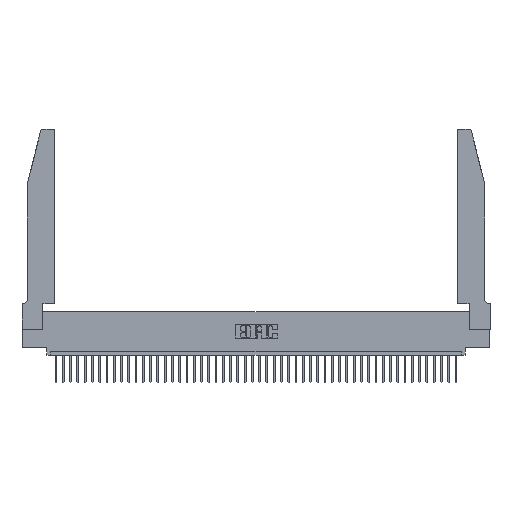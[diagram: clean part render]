
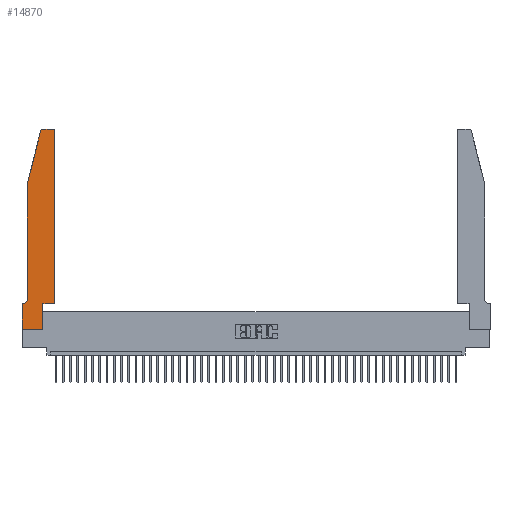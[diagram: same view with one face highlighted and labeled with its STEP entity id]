
A CAD part, top view. The second image highlights one B-rep face of the part: STEP entity #14870.
In plain terms, the highlighted planar face has unit normal (0, 0, 1).
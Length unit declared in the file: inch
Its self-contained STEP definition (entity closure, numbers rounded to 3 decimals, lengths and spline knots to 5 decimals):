
#922 = DIRECTION ( 'NONE',  ( 1., 0., 0. ) ) ;
#1242 = VERTEX_POINT ( 'NONE', #12942 ) ;
#1576 = DIRECTION ( 'NONE',  ( -1., 0., 0. ) ) ;
#1824 = VERTEX_POINT ( 'NONE', #16628 ) ;
#2136 = DIRECTION ( 'NONE',  ( -1., 0., 0. ) ) ;
#3395 = CIRCLE ( 'NONE', #24986, 0.03 ) ;
#4160 = ORIENTED_EDGE ( 'NONE', *, *, #15259, .T. ) ;
#4595 = LINE ( 'NONE', #15943, #15467 ) ;
#4754 = CARTESIAN_POINT ( 'NONE',  ( 0., 0.35, 0.37 ) ) ;
#4789 = EDGE_CURVE ( 'NONE', #6504, #27034, #36625, .T. ) ;
#5355 = ORIENTED_EDGE ( 'NONE', *, *, #10727, .T. ) ;
#5375 = VERTEX_POINT ( 'NONE', #40524 ) ;
#6130 = CARTESIAN_POINT ( 'NONE',  ( 0.0055, 0.42, 0.37 ) ) ;
#6171 = DIRECTION ( 'NONE',  ( 0., 1., 0. ) ) ;
#6495 = VECTOR ( 'NONE', #34825, 39.37008 ) ;
#6504 = VERTEX_POINT ( 'NONE', #4754 ) ;
#6997 = VERTEX_POINT ( 'NONE', #44194 ) ;
#7926 = EDGE_CURVE ( 'NONE', #5375, #38306, #26969, .T. ) ;
#9724 = CARTESIAN_POINT ( 'NONE',  ( 0., 0., 0.37 ) ) ;
#10621 = ORIENTED_EDGE ( 'NONE', *, *, #13284, .T. ) ;
#10727 = EDGE_CURVE ( 'NONE', #31694, #42694, #28785, .T. ) ;
#10803 = ORIENTED_EDGE ( 'NONE', *, *, #26341, .T. ) ;
#10925 = EDGE_CURVE ( 'NONE', #42694, #29869, #11331, .T. ) ;
#11331 = LINE ( 'NONE', #14977, #44713 ) ;
#11994 = AXIS2_PLACEMENT_3D ( 'NONE', #6130, #34358, #1576 ) ;
#12942 = CARTESIAN_POINT ( 'NONE',  ( 0.2865, 0., 0.37 ) ) ;
#13284 = EDGE_CURVE ( 'NONE', #20103, #5375, #24508, .T. ) ;
#14694 = VECTOR ( 'NONE', #44837, 39.37008 ) ;
#14740 = EDGE_CURVE ( 'NONE', #1242, #40147, #40765, .T. ) ;
#14870 = ADVANCED_FACE ( 'NONE', ( #26552 ), #24962, .T. ) ;
#14977 = CARTESIAN_POINT ( 'NONE',  ( 0.0755, 2., 0.37 ) ) ;
#15259 = EDGE_CURVE ( 'NONE', #27034, #1242, #40723, .T. ) ;
#15467 = VECTOR ( 'NONE', #23313, 39.37008 ) ;
#15488 = EDGE_CURVE ( 'NONE', #40147, #6997, #4595, .T. ) ;
#15943 = CARTESIAN_POINT ( 'NONE',  ( 0.4505, 0.35, 0.37 ) ) ;
#15975 = EDGE_LOOP ( 'NONE', ( #27805, #43039, #5355, #23073, #16473, #10803, #36767, #4160, #39724, #18869, #16064, #10621 ) ) ;
#16064 = ORIENTED_EDGE ( 'NONE', *, *, #36062, .T. ) ;
#16112 = CARTESIAN_POINT ( 'NONE',  ( 0.0755, 0.35, 0.37 ) ) ;
#16473 = ORIENTED_EDGE ( 'NONE', *, *, #17511, .T. ) ;
#16628 = CARTESIAN_POINT ( 'NONE',  ( 0.0055, 0.35, 0.37 ) ) ;
#16891 = AXIS2_PLACEMENT_3D ( 'NONE', #42460, #26202, #22196 ) ;
#17511 = EDGE_CURVE ( 'NONE', #29869, #1824, #23569, .T. ) ;
#18200 = DIRECTION ( 'NONE',  ( 1., 0., 0. ) ) ;
#18372 = CARTESIAN_POINT ( 'NONE',  ( 0.2865, 0.35, 0.37 ) ) ;
#18869 = ORIENTED_EDGE ( 'NONE', *, *, #15488, .T. ) ;
#20103 = VERTEX_POINT ( 'NONE', #31179 ) ;
#20938 = DIRECTION ( 'NONE',  ( 1., 0., 0. ) ) ;
#21409 = CARTESIAN_POINT ( 'NONE',  ( 0.0755, 0.42, 0.37 ) ) ;
#21632 = CARTESIAN_POINT ( 'NONE',  ( 0.25487, 2.72718, 0.37 ) ) ;
#22196 = DIRECTION ( 'NONE',  ( 1., 0., 0. ) ) ;
#23073 = ORIENTED_EDGE ( 'NONE', *, *, #10925, .T. ) ;
#23313 = DIRECTION ( 'NONE',  ( 1., 0., 0. ) ) ;
#23569 = CIRCLE ( 'NONE', #11994, 0.07 ) ;
#23901 = CARTESIAN_POINT ( 'NONE',  ( 0.4505, 0.35, 0.37 ) ) ;
#24457 = CARTESIAN_POINT ( 'NONE',  ( 0.284, 2.72, 0.37 ) ) ;
#24508 = CIRCLE ( 'NONE', #39127, 0.03 ) ;
#24962 = PLANE ( 'NONE',  #16891 ) ;
#24986 = AXIS2_PLACEMENT_3D ( 'NONE', #24457, #27948, #20938 ) ;
#26202 = DIRECTION ( 'NONE',  ( 0., 0., 1. ) ) ;
#26341 = EDGE_CURVE ( 'NONE', #1824, #6504, #43652, .T. ) ;
#26552 = FACE_OUTER_BOUND ( 'NONE', #15975, .T. ) ;
#26969 = LINE ( 'NONE', #33248, #43293 ) ;
#27034 = VERTEX_POINT ( 'NONE', #35215 ) ;
#27094 = CARTESIAN_POINT ( 'NONE',  ( 0.2865, 0.35, 0.37 ) ) ;
#27505 = CARTESIAN_POINT ( 'NONE',  ( 0.284, 2.75, 0.37 ) ) ;
#27521 = VECTOR ( 'NONE', #6171, 39.37008 ) ;
#27805 = ORIENTED_EDGE ( 'NONE', *, *, #7926, .T. ) ;
#27948 = DIRECTION ( 'NONE',  ( 0., 0., 1. ) ) ;
#28444 = DIRECTION ( 'NONE',  ( 0., 1., 0. ) ) ;
#28785 = LINE ( 'NONE', #31137, #6495 ) ;
#29869 = VERTEX_POINT ( 'NONE', #21409 ) ;
#31137 = CARTESIAN_POINT ( 'NONE',  ( 0.0755, 2., 0.37 ) ) ;
#31179 = CARTESIAN_POINT ( 'NONE',  ( 0.4505, 2.72, 0.37 ) ) ;
#31694 = VERTEX_POINT ( 'NONE', #21632 ) ;
#33248 = CARTESIAN_POINT ( 'NONE',  ( 0.2605, 2.75, 0.37 ) ) ;
#34358 = DIRECTION ( 'NONE',  ( 0., 0., -1. ) ) ;
#34825 = DIRECTION ( 'NONE',  ( -0.239, -0.971, 0. ) ) ;
#35215 = CARTESIAN_POINT ( 'NONE',  ( 0., 0., 0.37 ) ) ;
#36062 = EDGE_CURVE ( 'NONE', #6997, #20103, #36776, .T. ) ;
#36625 = LINE ( 'NONE', #9724, #14694 ) ;
#36629 = CARTESIAN_POINT ( 'NONE',  ( 0.0755, 2., 0.37 ) ) ;
#36767 = ORIENTED_EDGE ( 'NONE', *, *, #4789, .T. ) ;
#36776 = LINE ( 'NONE', #23901, #27521 ) ;
#37416 = VECTOR ( 'NONE', #18200, 39.37008 ) ;
#38306 = VERTEX_POINT ( 'NONE', #27505 ) ;
#38600 = CARTESIAN_POINT ( 'NONE',  ( 0.4205, 2.72, 0.37 ) ) ;
#39127 = AXIS2_PLACEMENT_3D ( 'NONE', #38600, #42704, #922 ) ;
#39416 = DIRECTION ( 'NONE',  ( 0., -1., 0. ) ) ;
#39724 = ORIENTED_EDGE ( 'NONE', *, *, #14740, .T. ) ;
#40147 = VERTEX_POINT ( 'NONE', #27094 ) ;
#40207 = VECTOR ( 'NONE', #28444, 39.37008 ) ;
#40524 = CARTESIAN_POINT ( 'NONE',  ( 0.4205, 2.75, 0.37 ) ) ;
#40723 = LINE ( 'NONE', #42587, #37416 ) ;
#40765 = LINE ( 'NONE', #18372, #40207 ) ;
#40959 = VECTOR ( 'NONE', #2136, 39.37008 ) ;
#42460 = CARTESIAN_POINT ( 'NONE',  ( 0., 0.35, 0.37 ) ) ;
#42587 = CARTESIAN_POINT ( 'NONE',  ( 0., 0., 0.37 ) ) ;
#42694 = VERTEX_POINT ( 'NONE', #36629 ) ;
#42704 = DIRECTION ( 'NONE',  ( 0., 0., 1. ) ) ;
#43039 = ORIENTED_EDGE ( 'NONE', *, *, #44186, .T. ) ;
#43293 = VECTOR ( 'NONE', #43472, 39.37008 ) ;
#43472 = DIRECTION ( 'NONE',  ( -1., 0., 0. ) ) ;
#43652 = LINE ( 'NONE', #16112, #40959 ) ;
#44186 = EDGE_CURVE ( 'NONE', #38306, #31694, #3395, .T. ) ;
#44194 = CARTESIAN_POINT ( 'NONE',  ( 0.4505, 0.35, 0.37 ) ) ;
#44713 = VECTOR ( 'NONE', #39416, 39.37008 ) ;
#44837 = DIRECTION ( 'NONE',  ( 0., -1., 0. ) ) ;
